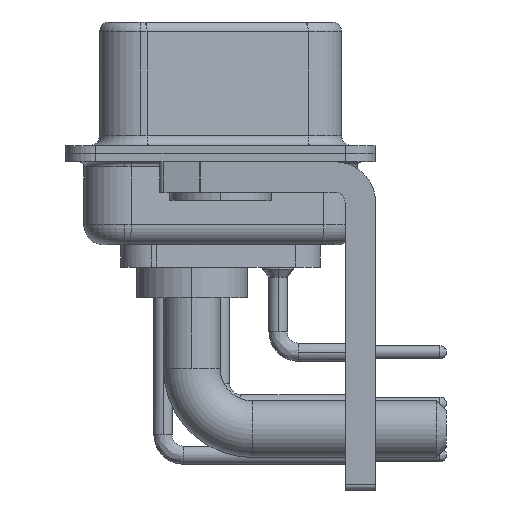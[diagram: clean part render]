
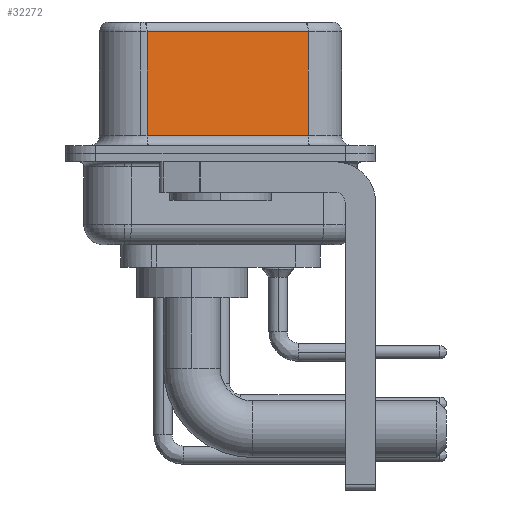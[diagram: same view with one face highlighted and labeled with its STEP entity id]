
A CAD part, left-side view. The second image highlights one B-rep face of the part: STEP entity #32272.
In plain terms, the highlighted planar face has unit normal (-0.985, -0.174, 0).
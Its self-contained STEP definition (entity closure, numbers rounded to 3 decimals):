
#575 = VERTEX_POINT ( 'NONE', #2370 ) ;
#1498 = ORIENTED_EDGE ( 'NONE', *, *, #3125, .T. ) ;
#1911 = VECTOR ( 'NONE', #31394, 1000. ) ;
#2238 = LINE ( 'NONE', #26175, #11702 ) ;
#2370 = CARTESIAN_POINT ( 'NONE',  ( 5.132, -4.322, 6.02 ) ) ;
#3125 = EDGE_CURVE ( 'NONE', #575, #10643, #12390, .T. ) ;
#4831 = ORIENTED_EDGE ( 'NONE', *, *, #27588, .T. ) ;
#5815 = LINE ( 'NONE', #27088, #33130 ) ;
#6870 = DIRECTION ( 'NONE',  ( -0.174, 0.985, 0. ) ) ;
#7056 = CARTESIAN_POINT ( 'NONE',  ( 3.73, 3.628, 6.02 ) ) ;
#7320 = LINE ( 'NONE', #23625, #1911 ) ;
#7913 = DIRECTION ( 'NONE',  ( 0.174, -0.985, 0. ) ) ;
#9004 = AXIS2_PLACEMENT_3D ( 'NONE', #13991, #24788, #11332 ) ;
#9282 = ORIENTED_EDGE ( 'NONE', *, *, #23569, .T. ) ;
#10643 = VERTEX_POINT ( 'NONE', #7056 ) ;
#11155 = CARTESIAN_POINT ( 'NONE',  ( 5.132, -4.322, 0.9 ) ) ;
#11332 = DIRECTION ( 'NONE',  ( -0.174, 0.985, 0. ) ) ;
#11702 = VECTOR ( 'NONE', #7913, 1000. ) ;
#12390 = LINE ( 'NONE', #14518, #30963 ) ;
#13991 = CARTESIAN_POINT ( 'NONE',  ( 5.132, -4.322, 6.52 ) ) ;
#14518 = CARTESIAN_POINT ( 'NONE',  ( 5.132, -4.322, 6.02 ) ) ;
#16182 = VERTEX_POINT ( 'NONE', #11155 ) ;
#18959 = CARTESIAN_POINT ( 'NONE',  ( 3.73, 3.628, 0.9 ) ) ;
#23569 = EDGE_CURVE ( 'NONE', #10643, #32090, #7320, .T. ) ;
#23625 = CARTESIAN_POINT ( 'NONE',  ( 3.73, 3.628, 6.52 ) ) ;
#24788 = DIRECTION ( 'NONE',  ( 0.985, 0.174, 0. ) ) ;
#26175 = CARTESIAN_POINT ( 'NONE',  ( 5.132, -4.322, 0.9 ) ) ;
#27088 = CARTESIAN_POINT ( 'NONE',  ( 5.132, -4.322, 6.52 ) ) ;
#27247 = EDGE_CURVE ( 'NONE', #575, #16182, #5815, .T. ) ;
#27451 = PLANE ( 'NONE',  #9004 ) ;
#27483 = EDGE_LOOP ( 'NONE', ( #28391, #1498, #9282, #4831 ) ) ;
#27588 = EDGE_CURVE ( 'NONE', #32090, #16182, #2238, .T. ) ;
#28391 = ORIENTED_EDGE ( 'NONE', *, *, #27247, .F. ) ;
#30420 = DIRECTION ( 'NONE',  ( 0., 0., -1. ) ) ;
#30963 = VECTOR ( 'NONE', #6870, 1000. ) ;
#31394 = DIRECTION ( 'NONE',  ( 0., 0., -1. ) ) ;
#32090 = VERTEX_POINT ( 'NONE', #18959 ) ;
#32272 = ADVANCED_FACE ( 'NONE', ( #32724 ), #27451, .F. ) ;
#32724 = FACE_OUTER_BOUND ( 'NONE', #27483, .T. ) ;
#33130 = VECTOR ( 'NONE', #30420, 1000. ) ;
